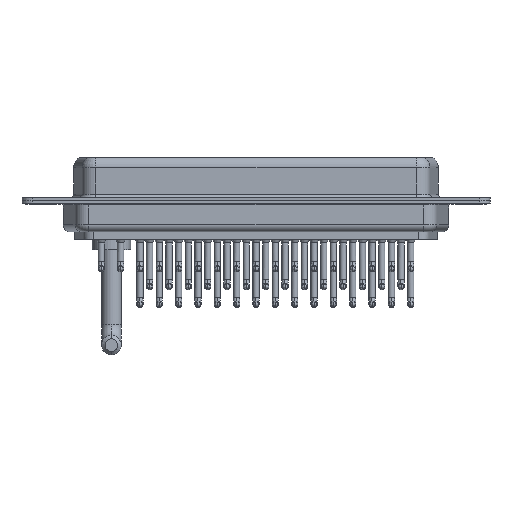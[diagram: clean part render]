
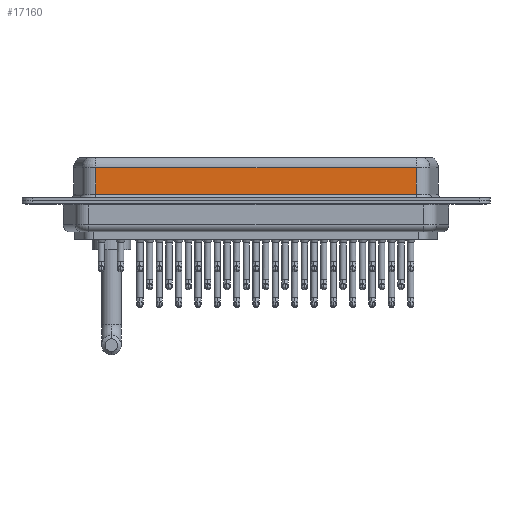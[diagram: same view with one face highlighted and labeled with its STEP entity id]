
A CAD part, front view. The second image highlights one B-rep face of the part: STEP entity #17160.
In plain terms, the highlighted planar face has unit normal (0, -1, 0).
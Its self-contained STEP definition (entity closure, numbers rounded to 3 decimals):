
#677 = LINE ( 'NONE', #13855, #29870 ) ;
#970 = CARTESIAN_POINT ( 'NONE',  ( 53.41, -5.375, 6.4 ) ) ;
#1491 = AXIS2_PLACEMENT_3D ( 'NONE', #18139, #15382, #11250 ) ;
#1757 = DIRECTION ( 'NONE',  ( -1., 0., 0. ) ) ;
#1920 = CARTESIAN_POINT ( 'NONE',  ( 53.41, -5.375, 4.65 ) ) ;
#2781 = EDGE_CURVE ( 'NONE', #6338, #27742, #677, .T. ) ;
#5914 = VECTOR ( 'NONE', #1757, 1000. ) ;
#6012 = LINE ( 'NONE', #970, #23210 ) ;
#6338 = VERTEX_POINT ( 'NONE', #20393 ) ;
#7105 = ORIENTED_EDGE ( 'NONE', *, *, #28389, .T. ) ;
#7305 = VERTEX_POINT ( 'NONE', #29420 ) ;
#10155 = PLANE ( 'NONE',  #1491 ) ;
#10213 = ORIENTED_EDGE ( 'NONE', *, *, #2781, .T. ) ;
#10230 = ORIENTED_EDGE ( 'NONE', *, *, #32034, .T. ) ;
#10655 = DIRECTION ( 'NONE',  ( 0., 0., -1. ) ) ;
#11215 = DIRECTION ( 'NONE',  ( 0., 0., -1. ) ) ;
#11250 = DIRECTION ( 'NONE',  ( 0., 0., 1. ) ) ;
#13550 = VECTOR ( 'NONE', #10655, 1000. ) ;
#13603 = CARTESIAN_POINT ( 'NONE',  ( 7.59, -5.375, 4.65 ) ) ;
#13855 = CARTESIAN_POINT ( 'NONE',  ( 53.41, -5.375, 0.9 ) ) ;
#13983 = EDGE_CURVE ( 'NONE', #7305, #27742, #6012, .T. ) ;
#15382 = DIRECTION ( 'NONE',  ( 0., 1., 0. ) ) ;
#16161 = VERTEX_POINT ( 'NONE', #13603 ) ;
#17160 = ADVANCED_FACE ( 'NONE', ( #27764 ), #10155, .F. ) ;
#18139 = CARTESIAN_POINT ( 'NONE',  ( 53.41, -5.375, 6.4 ) ) ;
#20393 = CARTESIAN_POINT ( 'NONE',  ( 7.59, -5.375, 0.9 ) ) ;
#21939 = LINE ( 'NONE', #1920, #5914 ) ;
#22713 = ORIENTED_EDGE ( 'NONE', *, *, #13983, .F. ) ;
#23210 = VECTOR ( 'NONE', #11215, 1000. ) ;
#24134 = CARTESIAN_POINT ( 'NONE',  ( 53.41, -5.375, 0.9 ) ) ;
#25495 = LINE ( 'NONE', #28409, #13550 ) ;
#25845 = EDGE_LOOP ( 'NONE', ( #22713, #10230, #7105, #10213 ) ) ;
#27742 = VERTEX_POINT ( 'NONE', #24134 ) ;
#27764 = FACE_OUTER_BOUND ( 'NONE', #25845, .T. ) ;
#28389 = EDGE_CURVE ( 'NONE', #16161, #6338, #25495, .T. ) ;
#28409 = CARTESIAN_POINT ( 'NONE',  ( 7.59, -5.375, 6.4 ) ) ;
#29420 = CARTESIAN_POINT ( 'NONE',  ( 53.41, -5.375, 4.65 ) ) ;
#29870 = VECTOR ( 'NONE', #31292, 1000. ) ;
#31292 = DIRECTION ( 'NONE',  ( 1., 0., 0. ) ) ;
#32034 = EDGE_CURVE ( 'NONE', #7305, #16161, #21939, .T. ) ;
